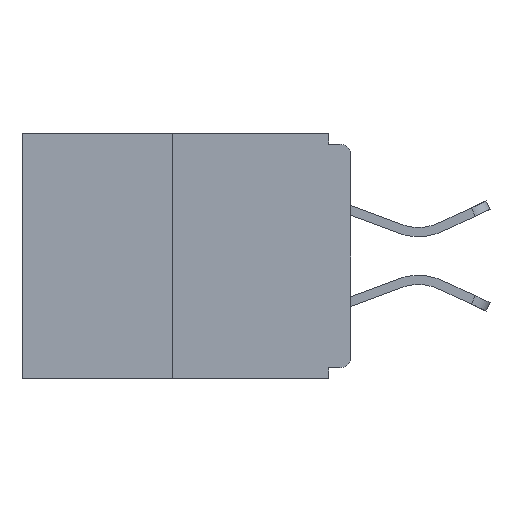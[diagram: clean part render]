
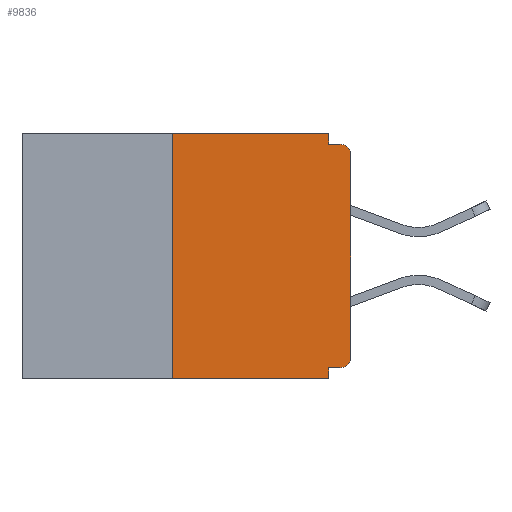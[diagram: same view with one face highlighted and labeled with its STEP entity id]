
A CAD part, left-side view. The second image highlights one B-rep face of the part: STEP entity #9836.
In plain terms, the highlighted planar face has unit normal (-1, 0, 0).
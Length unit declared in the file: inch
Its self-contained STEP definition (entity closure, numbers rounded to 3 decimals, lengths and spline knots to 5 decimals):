
#161 = DIRECTION ( 'NONE',  ( 0., 1., 0. ) ) ;
#212 = VERTEX_POINT ( 'NONE', #4119 ) ;
#239 = EDGE_CURVE ( 'NONE', #8344, #3884, #4513, .T. ) ;
#486 = ORIENTED_EDGE ( 'NONE', *, *, #8412, .T. ) ;
#566 = CARTESIAN_POINT ( 'NONE',  ( 0., 0.031, -0.343 ) ) ;
#614 = CARTESIAN_POINT ( 'NONE',  ( 0., 0.031, 0. ) ) ;
#760 = CARTESIAN_POINT ( 'NONE',  ( 0., 0.015, -0.328 ) ) ;
#930 = VECTOR ( 'NONE', #6361, 39.37008 ) ;
#1331 = EDGE_CURVE ( 'NONE', #7326, #5622, #12172, .T. ) ;
#1452 = VECTOR ( 'NONE', #10701, 39.37008 ) ;
#1741 = CARTESIAN_POINT ( 'NONE',  ( 0., 0., 0. ) ) ;
#1767 = CARTESIAN_POINT ( 'NONE',  ( 0., 0.25, -0.343 ) ) ;
#2163 = VECTOR ( 'NONE', #5295, 39.37008 ) ;
#2434 = LINE ( 'NONE', #4469, #8776 ) ;
#2459 = DIRECTION ( 'NONE',  ( 0., -1., 0. ) ) ;
#2572 = EDGE_CURVE ( 'NONE', #11166, #11100, #6180, .T. ) ;
#2820 = DIRECTION ( 'NONE',  ( -1., 0., 0. ) ) ;
#3233 = VERTEX_POINT ( 'NONE', #3257 ) ;
#3257 = CARTESIAN_POINT ( 'NONE',  ( 0., 0., -0.313 ) ) ;
#3329 = VECTOR ( 'NONE', #9739, 39.37008 ) ;
#3413 = EDGE_CURVE ( 'NONE', #5105, #5622, #12901, .T. ) ;
#3552 = PLANE ( 'NONE',  #8430 ) ;
#3884 = VERTEX_POINT ( 'NONE', #10893 ) ;
#4089 = ORIENTED_EDGE ( 'NONE', *, *, #11563, .F. ) ;
#4119 = CARTESIAN_POINT ( 'NONE',  ( 0., 0.031, -0.343 ) ) ;
#4324 = ORIENTED_EDGE ( 'NONE', *, *, #8194, .T. ) ;
#4469 = CARTESIAN_POINT ( 'NONE',  ( 0., 0.46, -0.343 ) ) ;
#4513 = LINE ( 'NONE', #6141, #2163 ) ;
#4916 = LINE ( 'NONE', #1741, #3329 ) ;
#5105 = VERTEX_POINT ( 'NONE', #10940 ) ;
#5107 = CARTESIAN_POINT ( 'NONE',  ( 0., 0.46, 0. ) ) ;
#5249 = ORIENTED_EDGE ( 'NONE', *, *, #2572, .F. ) ;
#5295 = DIRECTION ( 'NONE',  ( 0., 0., 1. ) ) ;
#5544 = CARTESIAN_POINT ( 'NONE',  ( 0., 0.015, -0.03 ) ) ;
#5586 = DIRECTION ( 'NONE',  ( 0., 0., -1. ) ) ;
#5622 = VERTEX_POINT ( 'NONE', #10562 ) ;
#5625 = CARTESIAN_POINT ( 'NONE',  ( 0., 0.031, -0.328 ) ) ;
#5924 = LINE ( 'NONE', #5107, #7846 ) ;
#6135 = CARTESIAN_POINT ( 'NONE',  ( 0., 0., -0.03 ) ) ;
#6141 = CARTESIAN_POINT ( 'NONE',  ( 0., 0.25, 0. ) ) ;
#6180 = LINE ( 'NONE', #11229, #7621 ) ;
#6361 = DIRECTION ( 'NONE',  ( 0., 0., -1. ) ) ;
#6719 = DIRECTION ( 'NONE',  ( 0., 0., -1. ) ) ;
#6808 = AXIS2_PLACEMENT_3D ( 'NONE', #5544, #11441, #5586 ) ;
#6913 = CARTESIAN_POINT ( 'NONE',  ( 0., 0., -0.015 ) ) ;
#7042 = DIRECTION ( 'NONE',  ( 0., -1., 0. ) ) ;
#7326 = VERTEX_POINT ( 'NONE', #6135 ) ;
#7506 = DIRECTION ( 'NONE',  ( 0., -1., 0. ) ) ;
#7621 = VECTOR ( 'NONE', #161, 39.37008 ) ;
#7846 = VECTOR ( 'NONE', #2459, 39.37008 ) ;
#7920 = VECTOR ( 'NONE', #7042, 39.37008 ) ;
#8099 = EDGE_LOOP ( 'NONE', ( #4089, #10544, #12897, #8327, #5249, #486, #4324, #10255, #9183, #8370 ) ) ;
#8194 = EDGE_CURVE ( 'NONE', #3233, #7326, #4916, .T. ) ;
#8327 = ORIENTED_EDGE ( 'NONE', *, *, #8584, .F. ) ;
#8341 = AXIS2_PLACEMENT_3D ( 'NONE', #10838, #2820, #12761 ) ;
#8344 = VERTEX_POINT ( 'NONE', #1767 ) ;
#8370 = ORIENTED_EDGE ( 'NONE', *, *, #9508, .F. ) ;
#8412 = EDGE_CURVE ( 'NONE', #11166, #3233, #12923, .T. ) ;
#8430 = AXIS2_PLACEMENT_3D ( 'NONE', #10718, #8740, #6719 ) ;
#8584 = EDGE_CURVE ( 'NONE', #11100, #212, #11368, .T. ) ;
#8740 = DIRECTION ( 'NONE',  ( 1., 0., 0. ) ) ;
#8776 = VECTOR ( 'NONE', #7506, 39.37008 ) ;
#9165 = FACE_OUTER_BOUND ( 'NONE', #8099, .T. ) ;
#9183 = ORIENTED_EDGE ( 'NONE', *, *, #3413, .F. ) ;
#9194 = VERTEX_POINT ( 'NONE', #614 ) ;
#9508 = EDGE_CURVE ( 'NONE', #9194, #5105, #12740, .T. ) ;
#9739 = DIRECTION ( 'NONE',  ( 0., 0., 1. ) ) ;
#9836 = ADVANCED_FACE ( 'NONE', ( #9165 ), #3552, .F. ) ;
#10255 = ORIENTED_EDGE ( 'NONE', *, *, #1331, .T. ) ;
#10544 = ORIENTED_EDGE ( 'NONE', *, *, #239, .F. ) ;
#10562 = CARTESIAN_POINT ( 'NONE',  ( 0., 0.015, -0.015 ) ) ;
#10701 = DIRECTION ( 'NONE',  ( 0., 0., -1. ) ) ;
#10718 = CARTESIAN_POINT ( 'NONE',  ( 0., 0.46, 0. ) ) ;
#10838 = CARTESIAN_POINT ( 'NONE',  ( 0., 0.015, -0.313 ) ) ;
#10893 = CARTESIAN_POINT ( 'NONE',  ( 0., 0.25, 0. ) ) ;
#10940 = CARTESIAN_POINT ( 'NONE',  ( 0., 0.031, -0.015 ) ) ;
#11100 = VERTEX_POINT ( 'NONE', #5625 ) ;
#11166 = VERTEX_POINT ( 'NONE', #760 ) ;
#11229 = CARTESIAN_POINT ( 'NONE',  ( 0., 0., -0.328 ) ) ;
#11368 = LINE ( 'NONE', #566, #1452 ) ;
#11386 = CARTESIAN_POINT ( 'NONE',  ( 0., 0.031, 0. ) ) ;
#11441 = DIRECTION ( 'NONE',  ( -1., 0., 0. ) ) ;
#11563 = EDGE_CURVE ( 'NONE', #3884, #9194, #5924, .T. ) ;
#12172 = CIRCLE ( 'NONE', #6808, 0.015 ) ;
#12552 = EDGE_CURVE ( 'NONE', #8344, #212, #2434, .T. ) ;
#12740 = LINE ( 'NONE', #11386, #930 ) ;
#12761 = DIRECTION ( 'NONE',  ( 0., 0., -1. ) ) ;
#12897 = ORIENTED_EDGE ( 'NONE', *, *, #12552, .T. ) ;
#12901 = LINE ( 'NONE', #6913, #7920 ) ;
#12923 = CIRCLE ( 'NONE', #8341, 0.015 ) ;
